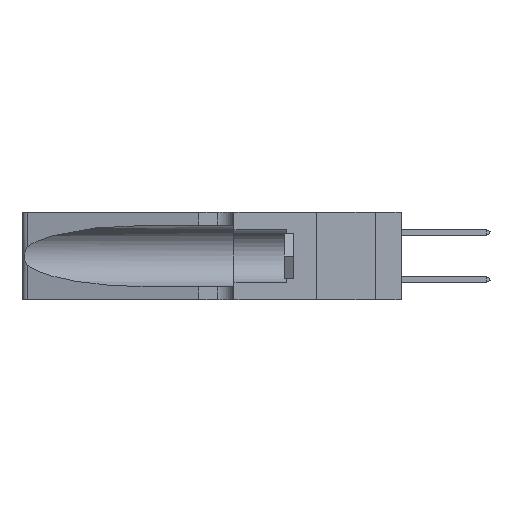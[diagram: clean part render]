
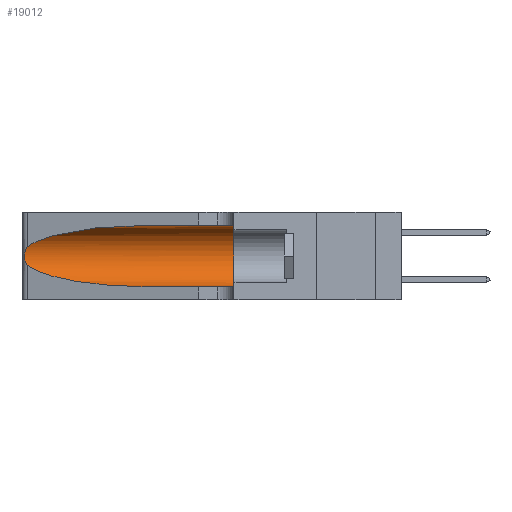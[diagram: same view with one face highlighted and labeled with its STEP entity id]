
A CAD part, left-side view. The second image highlights one B-rep face of the part: STEP entity #19012.
In plain terms, the highlighted cylindrical face has radius 3.308 mm (diameter 6.617 mm), a partial arc.
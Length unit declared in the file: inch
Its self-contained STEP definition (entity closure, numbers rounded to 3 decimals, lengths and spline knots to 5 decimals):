
#832 = DIRECTION ( 'NONE',  ( 0., -1., 0. ) ) ;
#901 = CARTESIAN_POINT ( 'NONE',  ( 0.25854, 1.2359, 0.20912 ) ) ;
#925 = CARTESIAN_POINT ( 'NONE',  ( 0.1305, 0.35, 0.31525 ) ) ;
#1114 = LINE ( 'NONE', #32481, #29535 ) ;
#3030 = AXIS2_PLACEMENT_3D ( 'NONE', #24253, #29397, #6801 ) ;
#3310 = CARTESIAN_POINT ( 'NONE',  ( 0.25639, 1.23186, 0.15144 ) ) ;
#3606 = CIRCLE ( 'NONE', #20049, 0.13025 ) ;
#3846 = CARTESIAN_POINT ( 'NONE',  ( 0.2373, 1.15595, 0.08982 ) ) ;
#3963 = CARTESIAN_POINT ( 'NONE',  ( 0.18966, 0.96281, 0.05475 ) ) ;
#4973 = ORIENTED_EDGE ( 'NONE', *, *, #29305, .T. ) ;
#5083 = EDGE_CURVE ( 'NONE', #7542, #6090, #3606, .T. ) ;
#5249 =( BOUNDED_CURVE ( )  B_SPLINE_CURVE ( 3, ( #23155, #23044, #15674, #5652 ),
 .UNSPECIFIED., .F., .T. ) 
 B_SPLINE_CURVE_WITH_KNOTS ( ( 4, 4 ),
 ( 1.5708, 2.84003 ),
 .UNSPECIFIED. ) 
 CURVE ( )  GEOMETRIC_REPRESENTATION_ITEM ( )  RATIONAL_B_SPLINE_CURVE ( ( 1., 0.87, 0.87, 1. ) ) 
 REPRESENTATION_ITEM ( '' )  );
#5652 = CARTESIAN_POINT ( 'NONE',  ( 0.25487, 1.22718, 0.22369 ) ) ;
#5761 = CARTESIAN_POINT ( 'NONE',  ( 0.26018, 1.23835, 0.19895 ) ) ;
#6083 = CARTESIAN_POINT ( 'NONE',  ( 0.26075, 1.23896, 0.178 ) ) ;
#6090 = VERTEX_POINT ( 'NONE', #9634 ) ;
#6401 = ORIENTED_EDGE ( 'NONE', *, *, #26888, .T. ) ;
#6414 = CARTESIAN_POINT ( 'NONE',  ( 0.25487, 1.22718, 0.22369 ) ) ;
#6801 = DIRECTION ( 'NONE',  ( 0., 0., -1. ) ) ;
#7542 = VERTEX_POINT ( 'NONE', #925 ) ;
#8515 = CARTESIAN_POINT ( 'NONE',  ( 0.1305, 0.72297, 0.31525 ) ) ;
#8624 = CARTESIAN_POINT ( 'NONE',  ( 0.25555, 1.22994, 0.2215 ) ) ;
#9634 = CARTESIAN_POINT ( 'NONE',  ( 0.1305, 0.35, 0.05475 ) ) ;
#12471 = DIRECTION ( 'NONE',  ( 0., -1., 0. ) ) ;
#12896 = EDGE_CURVE ( 'NONE', #16724, #7542, #1114, .T. ) ;
#13933 = ORIENTED_EDGE ( 'NONE', *, *, #5083, .F. ) ;
#15674 = CARTESIAN_POINT ( 'NONE',  ( 0.2373, 1.15595, 0.28018 ) ) ;
#15995 = CARTESIAN_POINT ( 'NONE',  ( 0.25789, 1.23486, 0.15765 ) ) ;
#16199 = CARTESIAN_POINT ( 'NONE',  ( 0.25555, 1.22993, 0.14849 ) ) ;
#16307 = CARTESIAN_POINT ( 'NONE',  ( 0.25487, 1.22718, 0.14631 ) ) ;
#16552 = CARTESIAN_POINT ( 'NONE',  ( 0.1305, 0.35, 0.185 ) ) ;
#16724 = VERTEX_POINT ( 'NONE', #8515 ) ;
#17215 = DIRECTION ( 'NONE',  ( 0., 1., 0. ) ) ;
#18433 = CARTESIAN_POINT ( 'NONE',  ( 0.25639, 1.23184, 0.21858 ) ) ;
#19012 = ADVANCED_FACE ( 'NONE', ( #20888 ), #19302, .F. ) ;
#19181 = CARTESIAN_POINT ( 'NONE',  ( 0.25487, 1.22718, 0.14631 ) ) ;
#19302 = CYLINDRICAL_SURFACE ( 'NONE', #3030, 0.13025 ) ;
#19847 = ORIENTED_EDGE ( 'NONE', *, *, #12896, .F. ) ;
#20049 = AXIS2_PLACEMENT_3D ( 'NONE', #16552, #17215, #22176 ) ;
#20529 =( BOUNDED_CURVE ( )  B_SPLINE_CURVE ( 3, ( #19181, #3846, #3963, #31212 ),
 .UNSPECIFIED., .F., .F. ) 
 B_SPLINE_CURVE_WITH_KNOTS ( ( 4, 4 ),
 ( 3.44316, 4.71239 ),
 .UNSPECIFIED. ) 
 CURVE ( )  GEOMETRIC_REPRESENTATION_ITEM ( )  RATIONAL_B_SPLINE_CURVE ( ( 1., 0.87, 0.87, 1. ) ) 
 REPRESENTATION_ITEM ( '' )  );
#20888 = FACE_OUTER_BOUND ( 'NONE', #27353, .T. ) ;
#20969 = CARTESIAN_POINT ( 'NONE',  ( 0.25787, 1.23484, 0.2124 ) ) ;
#22176 = DIRECTION ( 'NONE',  ( 0., 0., 1. ) ) ;
#22394 = ORIENTED_EDGE ( 'NONE', *, *, #29998, .T. ) ;
#23044 = CARTESIAN_POINT ( 'NONE',  ( 0.18966, 0.96281, 0.31525 ) ) ;
#23155 = CARTESIAN_POINT ( 'NONE',  ( 0.1305, 0.72297, 0.31525 ) ) ;
#23185 = VERTEX_POINT ( 'NONE', #30838 ) ;
#23460 = CARTESIAN_POINT ( 'NONE',  ( 0.26075, 1.23896, 0.19203 ) ) ;
#23717 = LINE ( 'NONE', #28624, #26484 ) ;
#24253 = CARTESIAN_POINT ( 'NONE',  ( 0.1305, 1.61858, 0.185 ) ) ;
#24806 = CARTESIAN_POINT ( 'NONE',  ( 0.1305, 0.72297, 0.05475 ) ) ;
#25918 = B_SPLINE_CURVE_WITH_KNOTS ( 'NONE', 3,
 ( #30898, #8624, #18433, #20969, #901, #5761, #23460, #6083, #25975, #31009, #15995, #3310, #16199, #16307 ),
 .UNSPECIFIED., .F., .F.,
 ( 4, 2, 2, 2, 2, 2, 4 ),
 ( 0., 0.00027, 0.00053, 0.00107, 0.0016, 0.00187, 0.00214 ),
 .UNSPECIFIED. ) ;
#25975 = CARTESIAN_POINT ( 'NONE',  ( 0.26017, 1.23833, 0.17102 ) ) ;
#26484 = VECTOR ( 'NONE', #832, 39.37008 ) ;
#26888 = EDGE_CURVE ( 'NONE', #23185, #31520, #20529, .T. ) ;
#27353 = EDGE_LOOP ( 'NONE', ( #30620, #22394, #6401, #4973, #13933, #19847 ) ) ;
#28624 = CARTESIAN_POINT ( 'NONE',  ( 0.1305, 1.61858, 0.05475 ) ) ;
#29305 = EDGE_CURVE ( 'NONE', #31520, #6090, #23717, .T. ) ;
#29397 = DIRECTION ( 'NONE',  ( 0., -1., 0. ) ) ;
#29535 = VECTOR ( 'NONE', #12471, 39.37008 ) ;
#29921 = EDGE_CURVE ( 'NONE', #16724, #30208, #5249, .T. ) ;
#29998 = EDGE_CURVE ( 'NONE', #30208, #23185, #25918, .T. ) ;
#30208 = VERTEX_POINT ( 'NONE', #6414 ) ;
#30620 = ORIENTED_EDGE ( 'NONE', *, *, #29921, .T. ) ;
#30838 = CARTESIAN_POINT ( 'NONE',  ( 0.25487, 1.22718, 0.14631 ) ) ;
#30898 = CARTESIAN_POINT ( 'NONE',  ( 0.25487, 1.22718, 0.22369 ) ) ;
#31009 = CARTESIAN_POINT ( 'NONE',  ( 0.25856, 1.23593, 0.16098 ) ) ;
#31212 = CARTESIAN_POINT ( 'NONE',  ( 0.1305, 0.72297, 0.05475 ) ) ;
#31520 = VERTEX_POINT ( 'NONE', #24806 ) ;
#32481 = CARTESIAN_POINT ( 'NONE',  ( 0.1305, 1.61858, 0.31525 ) ) ;
